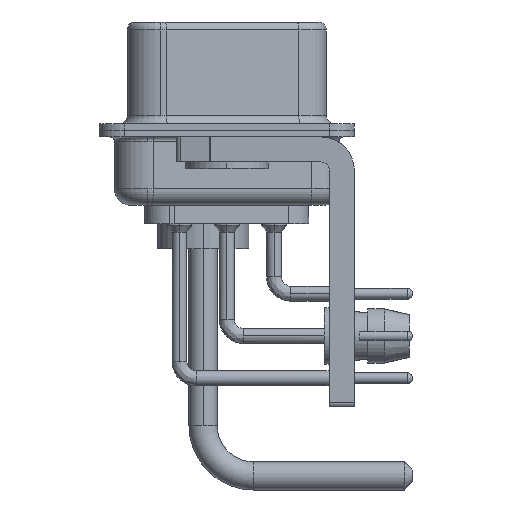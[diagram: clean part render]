
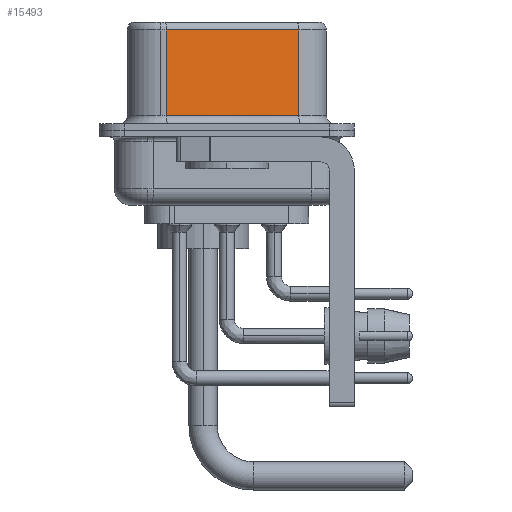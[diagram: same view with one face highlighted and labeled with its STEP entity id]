
A CAD part, left-side view. The second image highlights one B-rep face of the part: STEP entity #15493.
In plain terms, the highlighted planar face has unit normal (-0.985, -0.174, 0).
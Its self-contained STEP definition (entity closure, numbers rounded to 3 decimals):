
#1197 = FACE_OUTER_BOUND ( 'NONE', #15604, .T. ) ;
#1288 = VERTEX_POINT ( 'NONE', #2332 ) ;
#2332 = CARTESIAN_POINT ( 'NONE',  ( 3.73, 3.628, 0.9 ) ) ;
#3823 = VERTEX_POINT ( 'NONE', #37188 ) ;
#6614 = CARTESIAN_POINT ( 'NONE',  ( 5.132, -4.322, 0.9 ) ) ;
#6883 = DIRECTION ( 'NONE',  ( 0.985, 0.174, 0. ) ) ;
#7627 = ORIENTED_EDGE ( 'NONE', *, *, #38389, .T. ) ;
#7778 = EDGE_CURVE ( 'NONE', #30349, #9248, #20013, .T. ) ;
#9248 = VERTEX_POINT ( 'NONE', #38260 ) ;
#11159 = AXIS2_PLACEMENT_3D ( 'NONE', #34032, #6883, #18987 ) ;
#12846 = DIRECTION ( 'NONE',  ( 0.174, -0.985, 0. ) ) ;
#12960 = EDGE_CURVE ( 'NONE', #9248, #1288, #25167, .T. ) ;
#14406 = EDGE_CURVE ( 'NONE', #30349, #3823, #19362, .T. ) ;
#15493 = ADVANCED_FACE ( 'NONE', ( #1197 ), #31092, .F. ) ;
#15604 = EDGE_LOOP ( 'NONE', ( #23187, #33771, #32766, #7627 ) ) ;
#18945 = VECTOR ( 'NONE', #37102, 1000. ) ;
#18987 = DIRECTION ( 'NONE',  ( -0.174, 0.985, 0. ) ) ;
#19305 = VECTOR ( 'NONE', #29180, 1000. ) ;
#19362 = LINE ( 'NONE', #37535, #34005 ) ;
#20013 = LINE ( 'NONE', #25470, #19305 ) ;
#21440 = LINE ( 'NONE', #6614, #21804 ) ;
#21653 = CARTESIAN_POINT ( 'NONE',  ( 3.73, 3.628, 6.52 ) ) ;
#21804 = VECTOR ( 'NONE', #12846, 1000. ) ;
#23187 = ORIENTED_EDGE ( 'NONE', *, *, #14406, .F. ) ;
#25167 = LINE ( 'NONE', #21653, #18945 ) ;
#25470 = CARTESIAN_POINT ( 'NONE',  ( 5.132, -4.322, 6.02 ) ) ;
#27477 = CARTESIAN_POINT ( 'NONE',  ( 5.132, -4.322, 6.02 ) ) ;
#29180 = DIRECTION ( 'NONE',  ( -0.174, 0.985, 0. ) ) ;
#30349 = VERTEX_POINT ( 'NONE', #27477 ) ;
#31092 = PLANE ( 'NONE',  #11159 ) ;
#32766 = ORIENTED_EDGE ( 'NONE', *, *, #12960, .T. ) ;
#33771 = ORIENTED_EDGE ( 'NONE', *, *, #7778, .T. ) ;
#34005 = VECTOR ( 'NONE', #37732, 1000. ) ;
#34032 = CARTESIAN_POINT ( 'NONE',  ( 5.132, -4.322, 6.52 ) ) ;
#37102 = DIRECTION ( 'NONE',  ( 0., 0., -1. ) ) ;
#37188 = CARTESIAN_POINT ( 'NONE',  ( 5.132, -4.322, 0.9 ) ) ;
#37535 = CARTESIAN_POINT ( 'NONE',  ( 5.132, -4.322, 6.52 ) ) ;
#37732 = DIRECTION ( 'NONE',  ( 0., 0., -1. ) ) ;
#38260 = CARTESIAN_POINT ( 'NONE',  ( 3.73, 3.628, 6.02 ) ) ;
#38389 = EDGE_CURVE ( 'NONE', #1288, #3823, #21440, .T. ) ;
